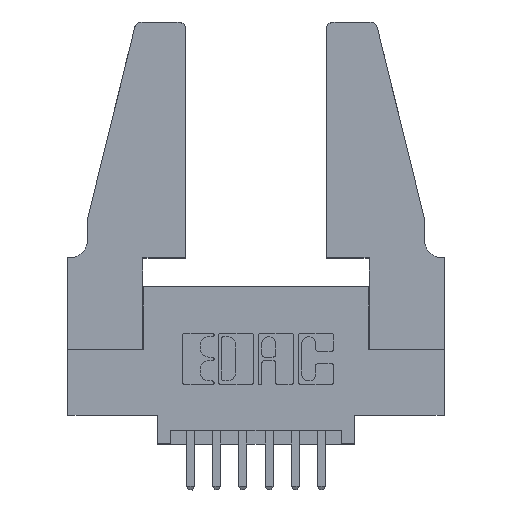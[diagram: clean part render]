
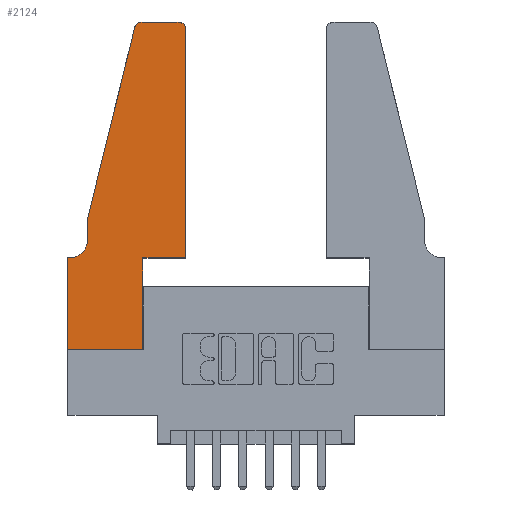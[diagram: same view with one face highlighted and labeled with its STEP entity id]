
A CAD part, top view. The second image highlights one B-rep face of the part: STEP entity #2124.
In plain terms, the highlighted planar face has unit normal (0, 0, 1).
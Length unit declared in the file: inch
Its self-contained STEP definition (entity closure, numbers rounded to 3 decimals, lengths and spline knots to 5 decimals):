
#124 = EDGE_CURVE ( 'NONE', #2681, #131, #7472, .T. ) ;
#131 = VERTEX_POINT ( 'NONE', #7013 ) ;
#254 = LINE ( 'NONE', #7919, #8885 ) ;
#263 = LINE ( 'NONE', #10722, #11534 ) ;
#340 = CARTESIAN_POINT ( 'NONE',  ( 0.0755, 0.35, 0.37 ) ) ;
#514 = CARTESIAN_POINT ( 'NONE',  ( 0.4505, 0.35, 0.37 ) ) ;
#574 = CARTESIAN_POINT ( 'NONE',  ( 0.4205, 1.22, 0.37 ) ) ;
#586 = ORIENTED_EDGE ( 'NONE', *, *, #1903, .T. ) ;
#728 = CARTESIAN_POINT ( 'NONE',  ( 0.2865, 0., 0.37 ) ) ;
#754 = ORIENTED_EDGE ( 'NONE', *, *, #4913, .T. ) ;
#882 = DIRECTION ( 'NONE',  ( -1., 0., 0. ) ) ;
#932 = VERTEX_POINT ( 'NONE', #3278 ) ;
#1193 = DIRECTION ( 'NONE',  ( 0., 0., 1. ) ) ;
#1197 = VERTEX_POINT ( 'NONE', #2907 ) ;
#1241 = CARTESIAN_POINT ( 'NONE',  ( 0.284, 1.22, 0.37 ) ) ;
#1275 = DIRECTION ( 'NONE',  ( 0., 1., 0. ) ) ;
#1283 = ORIENTED_EDGE ( 'NONE', *, *, #6808, .T. ) ;
#1330 = DIRECTION ( 'NONE',  ( -1., 0., 0. ) ) ;
#1466 = DIRECTION ( 'NONE',  ( 1., 0., 0. ) ) ;
#1484 = DIRECTION ( 'NONE',  ( 0., 0., 1. ) ) ;
#1503 = CARTESIAN_POINT ( 'NONE',  ( 0., 0.35, 0.37 ) ) ;
#1569 = CARTESIAN_POINT ( 'NONE',  ( 0.4505, 0.35, 0.37 ) ) ;
#1606 = ORIENTED_EDGE ( 'NONE', *, *, #9758, .T. ) ;
#1620 = CARTESIAN_POINT ( 'NONE',  ( 0.2605, 1.25, 0.37 ) ) ;
#1891 = CARTESIAN_POINT ( 'NONE',  ( 0.0055, 0.35, 0.37 ) ) ;
#1903 = EDGE_CURVE ( 'NONE', #8778, #9325, #5451, .T. ) ;
#2039 = ORIENTED_EDGE ( 'NONE', *, *, #2160, .T. ) ;
#2049 = VECTOR ( 'NONE', #3453, 39.37008 ) ;
#2124 = ADVANCED_FACE ( 'NONE', ( #10946 ), #5175, .T. ) ;
#2160 = EDGE_CURVE ( 'NONE', #4369, #1197, #5605, .T. ) ;
#2171 = CARTESIAN_POINT ( 'NONE',  ( 0., 0.35, 0.37 ) ) ;
#2466 = CARTESIAN_POINT ( 'NONE',  ( 0.25487, 1.22718, 0.37 ) ) ;
#2657 = DIRECTION ( 'NONE',  ( -1., 0., 0. ) ) ;
#2681 = VERTEX_POINT ( 'NONE', #11059 ) ;
#2693 = ORIENTED_EDGE ( 'NONE', *, *, #10636, .T. ) ;
#2695 = DIRECTION ( 'NONE',  ( -0.239, -0.971, 0. ) ) ;
#2907 = CARTESIAN_POINT ( 'NONE',  ( 0.2865, 0.35, 0.37 ) ) ;
#2956 = EDGE_CURVE ( 'NONE', #131, #7831, #3539, .T. ) ;
#3278 = CARTESIAN_POINT ( 'NONE',  ( 0., 0., 0.37 ) ) ;
#3418 = CARTESIAN_POINT ( 'NONE',  ( 0.284, 1.25, 0.37 ) ) ;
#3453 = DIRECTION ( 'NONE',  ( 0., 1., 0. ) ) ;
#3539 = LINE ( 'NONE', #1620, #4254 ) ;
#3854 = CARTESIAN_POINT ( 'NONE',  ( 0.0055, 0.42, 0.37 ) ) ;
#4244 = VERTEX_POINT ( 'NONE', #5759 ) ;
#4254 = VECTOR ( 'NONE', #882, 39.37008 ) ;
#4322 = EDGE_CURVE ( 'NONE', #9511, #932, #6402, .T. ) ;
#4325 = ORIENTED_EDGE ( 'NONE', *, *, #124, .T. ) ;
#4369 = VERTEX_POINT ( 'NONE', #728 ) ;
#4657 = VECTOR ( 'NONE', #2695, 39.37008 ) ;
#4913 = EDGE_CURVE ( 'NONE', #7191, #4244, #10428, .T. ) ;
#5023 = AXIS2_PLACEMENT_3D ( 'NONE', #574, #1484, #8830 ) ;
#5109 = DIRECTION ( 'NONE',  ( 0., -1., 0. ) ) ;
#5175 = PLANE ( 'NONE',  #7713 ) ;
#5353 = VECTOR ( 'NONE', #1466, 39.37008 ) ;
#5451 = CIRCLE ( 'NONE', #6857, 0.07 ) ;
#5487 = EDGE_CURVE ( 'NONE', #9325, #9511, #10570, .T. ) ;
#5526 = DIRECTION ( 'NONE',  ( 0., 0., -1. ) ) ;
#5605 = LINE ( 'NONE', #11522, #7000 ) ;
#5688 = VECTOR ( 'NONE', #5109, 39.37008 ) ;
#5759 = CARTESIAN_POINT ( 'NONE',  ( 0.0755, 0.5, 0.37 ) ) ;
#5874 = AXIS2_PLACEMENT_3D ( 'NONE', #1241, #1193, #7615 ) ;
#6029 = VERTEX_POINT ( 'NONE', #6261 ) ;
#6174 = DIRECTION ( 'NONE',  ( 1., 0., 0. ) ) ;
#6261 = CARTESIAN_POINT ( 'NONE',  ( 0.4505, 0.35, 0.37 ) ) ;
#6402 = LINE ( 'NONE', #7046, #5688 ) ;
#6412 = CARTESIAN_POINT ( 'NONE',  ( 0.0755, 0.42, 0.37 ) ) ;
#6535 = EDGE_CURVE ( 'NONE', #6029, #2681, #6911, .T. ) ;
#6808 = EDGE_CURVE ( 'NONE', #1197, #6029, #11143, .T. ) ;
#6812 = ORIENTED_EDGE ( 'NONE', *, *, #5487, .T. ) ;
#6857 = AXIS2_PLACEMENT_3D ( 'NONE', #3854, #5526, #2657 ) ;
#6911 = LINE ( 'NONE', #1569, #2049 ) ;
#7000 = VECTOR ( 'NONE', #1275, 39.37008 ) ;
#7013 = CARTESIAN_POINT ( 'NONE',  ( 0.4205, 1.25, 0.37 ) ) ;
#7046 = CARTESIAN_POINT ( 'NONE',  ( 0., 0., 0.37 ) ) ;
#7103 = CARTESIAN_POINT ( 'NONE',  ( 0.0755, 0.5, 0.37 ) ) ;
#7107 = EDGE_LOOP ( 'NONE', ( #7391, #1606, #754, #10348, #586, #6812, #11466, #2693, #2039, #1283, #7809, #4325 ) ) ;
#7191 = VERTEX_POINT ( 'NONE', #2466 ) ;
#7391 = ORIENTED_EDGE ( 'NONE', *, *, #2956, .T. ) ;
#7472 = CIRCLE ( 'NONE', #5023, 0.03 ) ;
#7615 = DIRECTION ( 'NONE',  ( 1., 0., 0. ) ) ;
#7713 = AXIS2_PLACEMENT_3D ( 'NONE', #1503, #9792, #10743 ) ;
#7809 = ORIENTED_EDGE ( 'NONE', *, *, #6535, .T. ) ;
#7831 = VERTEX_POINT ( 'NONE', #3418 ) ;
#7919 = CARTESIAN_POINT ( 'NONE',  ( 0., 0., 0.37 ) ) ;
#8117 = EDGE_CURVE ( 'NONE', #4244, #8778, #263, .T. ) ;
#8778 = VERTEX_POINT ( 'NONE', #6412 ) ;
#8830 = DIRECTION ( 'NONE',  ( 1., 0., 0. ) ) ;
#8885 = VECTOR ( 'NONE', #6174, 39.37008 ) ;
#9325 = VERTEX_POINT ( 'NONE', #1891 ) ;
#9511 = VERTEX_POINT ( 'NONE', #2171 ) ;
#9649 = CIRCLE ( 'NONE', #5874, 0.03 ) ;
#9758 = EDGE_CURVE ( 'NONE', #7831, #7191, #9649, .T. ) ;
#9792 = DIRECTION ( 'NONE',  ( 0., 0., 1. ) ) ;
#9816 = DIRECTION ( 'NONE',  ( 0., -1., 0. ) ) ;
#10348 = ORIENTED_EDGE ( 'NONE', *, *, #8117, .T. ) ;
#10428 = LINE ( 'NONE', #7103, #4657 ) ;
#10570 = LINE ( 'NONE', #340, #10887 ) ;
#10636 = EDGE_CURVE ( 'NONE', #932, #4369, #254, .T. ) ;
#10722 = CARTESIAN_POINT ( 'NONE',  ( 0.0755, 0.5, 0.37 ) ) ;
#10743 = DIRECTION ( 'NONE',  ( 1., 0., 0. ) ) ;
#10887 = VECTOR ( 'NONE', #1330, 39.37008 ) ;
#10946 = FACE_OUTER_BOUND ( 'NONE', #7107, .T. ) ;
#11059 = CARTESIAN_POINT ( 'NONE',  ( 0.4505, 1.22, 0.37 ) ) ;
#11143 = LINE ( 'NONE', #514, #5353 ) ;
#11466 = ORIENTED_EDGE ( 'NONE', *, *, #4322, .T. ) ;
#11522 = CARTESIAN_POINT ( 'NONE',  ( 0.2865, 0.35, 0.37 ) ) ;
#11534 = VECTOR ( 'NONE', #9816, 39.37008 ) ;
